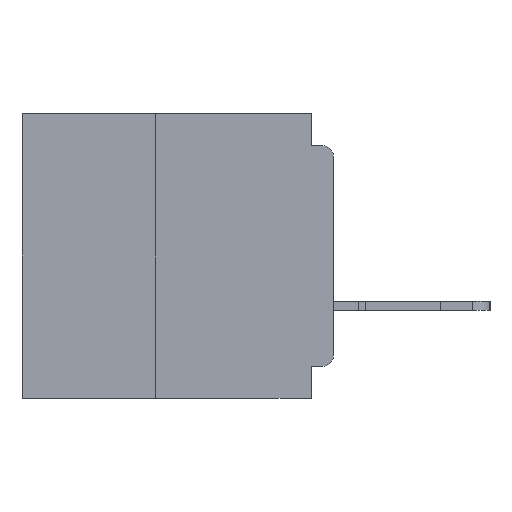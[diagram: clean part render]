
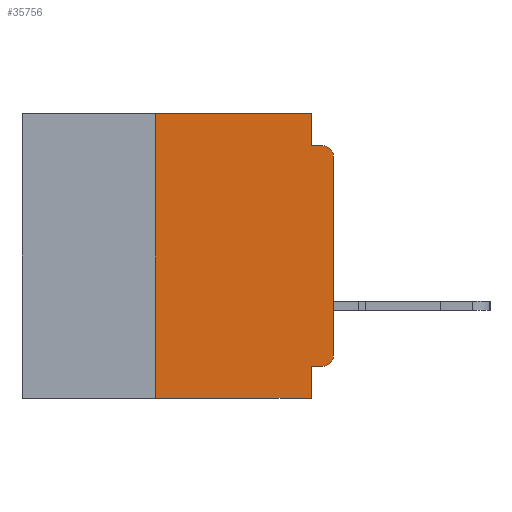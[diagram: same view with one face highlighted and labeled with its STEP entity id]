
A CAD part, left-side view. The second image highlights one B-rep face of the part: STEP entity #35756.
In plain terms, the highlighted planar face has unit normal (-1, 0, 0).
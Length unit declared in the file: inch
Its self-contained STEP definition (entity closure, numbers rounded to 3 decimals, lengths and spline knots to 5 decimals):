
#1424 = VECTOR ( 'NONE', #31444, 39.37008 ) ;
#2475 = CARTESIAN_POINT ( 'NONE',  ( 0., 0.031, 0. ) ) ;
#2627 = VERTEX_POINT ( 'NONE', #30396 ) ;
#3085 = EDGE_LOOP ( 'NONE', ( #33319, #32985, #46171, #45768, #24372, #15866, #14983, #15932, #22680, #22739 ) ) ;
#3427 = CARTESIAN_POINT ( 'NONE',  ( 0., 0., -0.355 ) ) ;
#3633 = AXIS2_PLACEMENT_3D ( 'NONE', #23752, #55886, #28489 ) ;
#4274 = VERTEX_POINT ( 'NONE', #7538 ) ;
#4569 = CIRCLE ( 'NONE', #3633, 0.015 ) ;
#5583 = VECTOR ( 'NONE', #32960, 39.37008 ) ;
#7306 = LINE ( 'NONE', #47157, #55059 ) ;
#7340 = LINE ( 'NONE', #56853, #55092 ) ;
#7538 = CARTESIAN_POINT ( 'NONE',  ( 0., 0.015, -0.355 ) ) ;
#7760 = CARTESIAN_POINT ( 'NONE',  ( 0., 0.031, -0.045 ) ) ;
#8714 = CARTESIAN_POINT ( 'NONE',  ( 0., 0., -0.045 ) ) ;
#8972 = CARTESIAN_POINT ( 'NONE',  ( 0., 0.437, 0. ) ) ;
#9921 = CARTESIAN_POINT ( 'NONE',  ( 0., 0.031, -0.355 ) ) ;
#9925 = EDGE_CURVE ( 'NONE', #37400, #46126, #11829, .T. ) ;
#10736 = EDGE_CURVE ( 'NONE', #39436, #50301, #22661, .T. ) ;
#11829 = LINE ( 'NONE', #8714, #55118 ) ;
#13731 = DIRECTION ( 'NONE',  ( 0., 0., -1. ) ) ;
#13912 = EDGE_CURVE ( 'NONE', #4274, #26472, #59491, .T. ) ;
#14810 = CARTESIAN_POINT ( 'NONE',  ( 0., 0.031, -0.4 ) ) ;
#14983 = ORIENTED_EDGE ( 'NONE', *, *, #31331, .T. ) ;
#15866 = ORIENTED_EDGE ( 'NONE', *, *, #56791, .F. ) ;
#15894 = DIRECTION ( 'NONE',  ( -1., 0., 0. ) ) ;
#15932 = ORIENTED_EDGE ( 'NONE', *, *, #10736, .F. ) ;
#16467 = LINE ( 'NONE', #41607, #51864 ) ;
#17884 = CARTESIAN_POINT ( 'NONE',  ( 0., 0., -0.06 ) ) ;
#18114 = EDGE_CURVE ( 'NONE', #26472, #47523, #30510, .T. ) ;
#19298 = FACE_OUTER_BOUND ( 'NONE', #3085, .T. ) ;
#22030 = AXIS2_PLACEMENT_3D ( 'NONE', #8972, #41552, #13731 ) ;
#22661 = LINE ( 'NONE', #51757, #59248 ) ;
#22680 = ORIENTED_EDGE ( 'NONE', *, *, #46858, .F. ) ;
#22739 = ORIENTED_EDGE ( 'NONE', *, *, #13912, .T. ) ;
#23038 = AXIS2_PLACEMENT_3D ( 'NONE', #43682, #15894, #48267 ) ;
#23752 = CARTESIAN_POINT ( 'NONE',  ( 0., 0.015, -0.06 ) ) ;
#24372 = ORIENTED_EDGE ( 'NONE', *, *, #46777, .F. ) ;
#24825 = CARTESIAN_POINT ( 'NONE',  ( 0., 0.031, 0. ) ) ;
#26472 = VERTEX_POINT ( 'NONE', #47107 ) ;
#28285 = CARTESIAN_POINT ( 'NONE',  ( 0., 0., 0. ) ) ;
#28489 = DIRECTION ( 'NONE',  ( 0., 0., -1. ) ) ;
#29429 = CARTESIAN_POINT ( 'NONE',  ( 0., 0.25, 0. ) ) ;
#30396 = CARTESIAN_POINT ( 'NONE',  ( 0., 0.25, -0.4 ) ) ;
#30510 = LINE ( 'NONE', #28285, #5583 ) ;
#31331 = EDGE_CURVE ( 'NONE', #2627, #50301, #7340, .T. ) ;
#31444 = DIRECTION ( 'NONE',  ( 0., 1., 0. ) ) ;
#32584 = CARTESIAN_POINT ( 'NONE',  ( 0., 0.015, -0.045 ) ) ;
#32952 = EDGE_CURVE ( 'NONE', #36577, #37400, #36331, .T. ) ;
#32960 = DIRECTION ( 'NONE',  ( 0., 0., 1. ) ) ;
#32985 = ORIENTED_EDGE ( 'NONE', *, *, #37027, .T. ) ;
#33319 = ORIENTED_EDGE ( 'NONE', *, *, #18114, .T. ) ;
#33554 = DIRECTION ( 'NONE',  ( 0., 0., -1. ) ) ;
#35756 = ADVANCED_FACE ( 'NONE', ( #19298 ), #36934, .F. ) ;
#35966 = VERTEX_POINT ( 'NONE', #29429 ) ;
#36331 = LINE ( 'NONE', #2475, #59108 ) ;
#36577 = VERTEX_POINT ( 'NONE', #24825 ) ;
#36689 = DIRECTION ( 'NONE',  ( 0., -1., 0. ) ) ;
#36934 = PLANE ( 'NONE',  #22030 ) ;
#37027 = EDGE_CURVE ( 'NONE', #47523, #46126, #4569, .T. ) ;
#37400 = VERTEX_POINT ( 'NONE', #7760 ) ;
#39436 = VERTEX_POINT ( 'NONE', #9921 ) ;
#39774 = DIRECTION ( 'NONE',  ( 0., 0., -1. ) ) ;
#41552 = DIRECTION ( 'NONE',  ( 1., 0., 0. ) ) ;
#41607 = CARTESIAN_POINT ( 'NONE',  ( 0., 0.25, -0.4 ) ) ;
#43682 = CARTESIAN_POINT ( 'NONE',  ( 0., 0.015, -0.34 ) ) ;
#45768 = ORIENTED_EDGE ( 'NONE', *, *, #32952, .F. ) ;
#46126 = VERTEX_POINT ( 'NONE', #32584 ) ;
#46171 = ORIENTED_EDGE ( 'NONE', *, *, #9925, .F. ) ;
#46777 = EDGE_CURVE ( 'NONE', #35966, #36577, #7306, .T. ) ;
#46858 = EDGE_CURVE ( 'NONE', #4274, #39436, #50809, .T. ) ;
#47107 = CARTESIAN_POINT ( 'NONE',  ( 0., 0., -0.34 ) ) ;
#47157 = CARTESIAN_POINT ( 'NONE',  ( 0., 0.437, 0. ) ) ;
#47523 = VERTEX_POINT ( 'NONE', #17884 ) ;
#48267 = DIRECTION ( 'NONE',  ( 0., 0., -1. ) ) ;
#50301 = VERTEX_POINT ( 'NONE', #14810 ) ;
#50770 = DIRECTION ( 'NONE',  ( 0., 0., 1. ) ) ;
#50809 = LINE ( 'NONE', #3427, #1424 ) ;
#51727 = DIRECTION ( 'NONE',  ( 0., -1., 0. ) ) ;
#51757 = CARTESIAN_POINT ( 'NONE',  ( 0., 0.031, -0.4 ) ) ;
#51864 = VECTOR ( 'NONE', #50770, 39.37008 ) ;
#55059 = VECTOR ( 'NONE', #51727, 39.37008 ) ;
#55092 = VECTOR ( 'NONE', #57037, 39.37008 ) ;
#55118 = VECTOR ( 'NONE', #36689, 39.37008 ) ;
#55886 = DIRECTION ( 'NONE',  ( -1., 0., 0. ) ) ;
#56791 = EDGE_CURVE ( 'NONE', #2627, #35966, #16467, .T. ) ;
#56853 = CARTESIAN_POINT ( 'NONE',  ( 0., 0.437, -0.4 ) ) ;
#57037 = DIRECTION ( 'NONE',  ( 0., -1., 0. ) ) ;
#59108 = VECTOR ( 'NONE', #39774, 39.37008 ) ;
#59248 = VECTOR ( 'NONE', #33554, 39.37008 ) ;
#59491 = CIRCLE ( 'NONE', #23038, 0.015 ) ;
